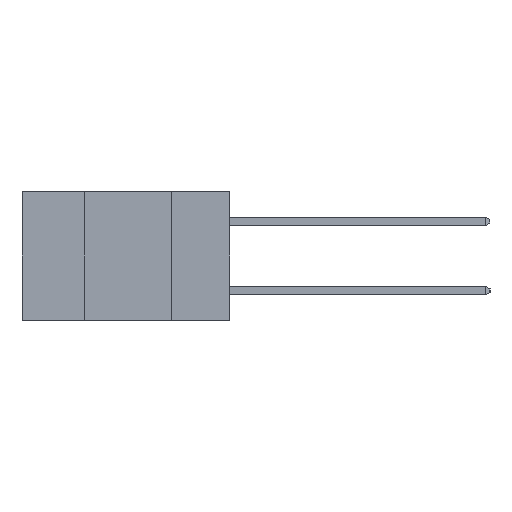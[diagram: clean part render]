
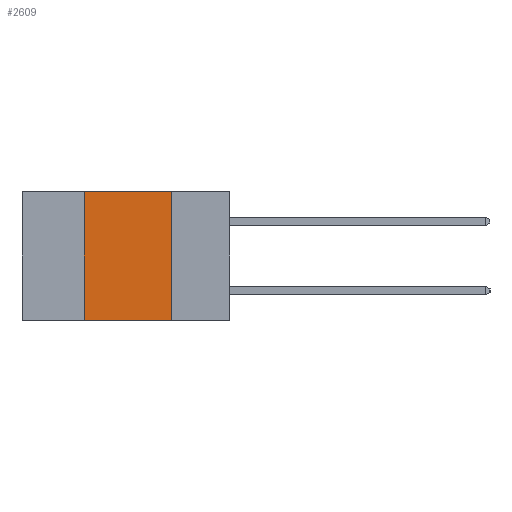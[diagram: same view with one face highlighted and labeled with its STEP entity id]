
A CAD part, left-side view. The second image highlights one B-rep face of the part: STEP entity #2609.
In plain terms, the highlighted planar face has unit normal (-1, 0, 0).
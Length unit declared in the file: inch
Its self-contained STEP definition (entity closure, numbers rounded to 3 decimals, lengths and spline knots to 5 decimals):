
#1192 = VERTEX_POINT ( 'NONE', #22810 ) ;
#2609 = ADVANCED_FACE ( 'NONE', ( #6391 ), #17005, .F. ) ;
#3905 = DIRECTION ( 'NONE',  ( 0., 0., -1. ) ) ;
#4627 = EDGE_CURVE ( 'NONE', #7049, #1192, #6590, .T. ) ;
#5010 = CARTESIAN_POINT ( 'NONE',  ( 0., 0.42, 0. ) ) ;
#5110 = EDGE_CURVE ( 'NONE', #24261, #17223, #20347, .T. ) ;
#5266 = CARTESIAN_POINT ( 'NONE',  ( 0., 0.17, 0. ) ) ;
#5666 = VECTOR ( 'NONE', #8549, 39.37008 ) ;
#5953 = ORIENTED_EDGE ( 'NONE', *, *, #8802, .F. ) ;
#6391 = FACE_OUTER_BOUND ( 'NONE', #19944, .T. ) ;
#6590 = LINE ( 'NONE', #13229, #22183 ) ;
#7049 = VERTEX_POINT ( 'NONE', #24197 ) ;
#8549 = DIRECTION ( 'NONE',  ( 0., 0., 1. ) ) ;
#8802 = EDGE_CURVE ( 'NONE', #7049, #24261, #20669, .T. ) ;
#9149 = EDGE_CURVE ( 'NONE', #17223, #1192, #23045, .T. ) ;
#9914 = ORIENTED_EDGE ( 'NONE', *, *, #5110, .F. ) ;
#13229 = CARTESIAN_POINT ( 'NONE',  ( 0., 0.6, -0.37 ) ) ;
#13313 = DIRECTION ( 'NONE',  ( 0., -1., 0. ) ) ;
#14639 = ORIENTED_EDGE ( 'NONE', *, *, #4627, .T. ) ;
#15157 = VECTOR ( 'NONE', #20476, 39.37008 ) ;
#15481 = AXIS2_PLACEMENT_3D ( 'NONE', #17116, #16955, #16926 ) ;
#16926 = DIRECTION ( 'NONE',  ( 0., 0., -1. ) ) ;
#16955 = DIRECTION ( 'NONE',  ( 1., 0., 0. ) ) ;
#17005 = PLANE ( 'NONE',  #15481 ) ;
#17116 = CARTESIAN_POINT ( 'NONE',  ( 0., 0.6, 0. ) ) ;
#17223 = VERTEX_POINT ( 'NONE', #5266 ) ;
#17629 = CARTESIAN_POINT ( 'NONE',  ( 0., 0.17, -0.37 ) ) ;
#17919 = VECTOR ( 'NONE', #3905, 39.37008 ) ;
#18525 = CARTESIAN_POINT ( 'NONE',  ( 0., 0.6, 0. ) ) ;
#19944 = EDGE_LOOP ( 'NONE', ( #24251, #9914, #5953, #14639 ) ) ;
#20265 = CARTESIAN_POINT ( 'NONE',  ( 0., 0.42, -0.37 ) ) ;
#20347 = LINE ( 'NONE', #18525, #15157 ) ;
#20476 = DIRECTION ( 'NONE',  ( 0., -1., 0. ) ) ;
#20669 = LINE ( 'NONE', #20265, #5666 ) ;
#22183 = VECTOR ( 'NONE', #13313, 39.37008 ) ;
#22810 = CARTESIAN_POINT ( 'NONE',  ( 0., 0.17, -0.37 ) ) ;
#23045 = LINE ( 'NONE', #17629, #17919 ) ;
#24197 = CARTESIAN_POINT ( 'NONE',  ( 0., 0.42, -0.37 ) ) ;
#24251 = ORIENTED_EDGE ( 'NONE', *, *, #9149, .F. ) ;
#24261 = VERTEX_POINT ( 'NONE', #5010 ) ;
